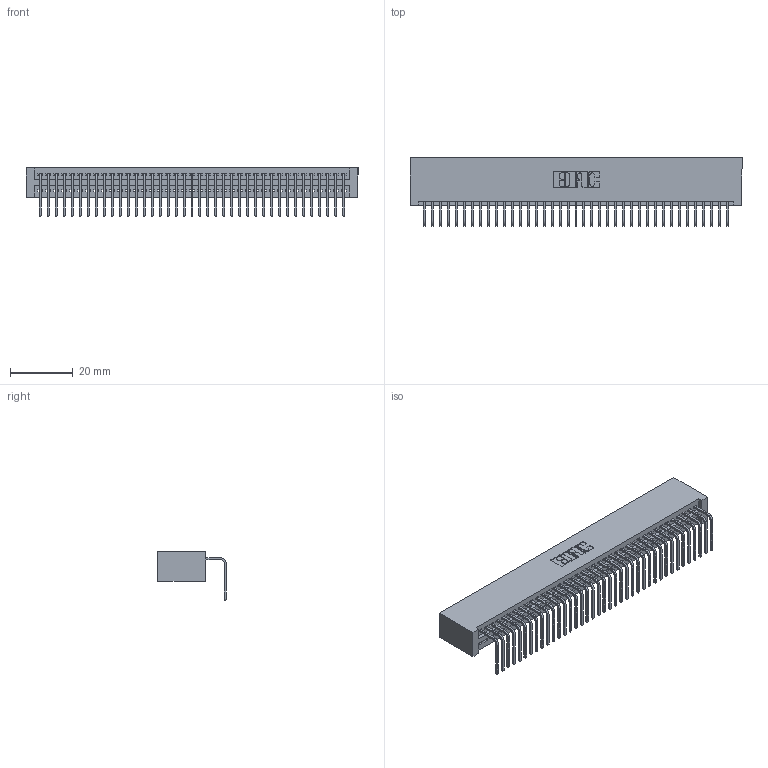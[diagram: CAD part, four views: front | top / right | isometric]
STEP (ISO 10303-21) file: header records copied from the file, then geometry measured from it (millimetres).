
FILE_DESCRIPTION (( 'STEP AP203' ), '1' );
FILE_NAME ('345-039-558-101.STEP', '2019-10-10T15:48:00', ( '' ), ( '' ), 'SwSTEP 2.0', 'SolidWorks 2016', '' );
FILE_SCHEMA (( 'CONFIG_CONTROL_DESIGN' ));
Length unit declared in the file: inch
Products named in the file (3): 345-039-558-101; 345 Part_No Mounting Lugs; 345-292-001_558 Tail - 2
Assembly tree (40 placements, depth 2):
  345-039-558-101
    345 Part_No Mounting Lugs
    345-292-001_558 Tail - 2  x39
Bounding box: 105.66 x 21.83 x 15.37 mm (x, y, z)
Volume: 10725.8 mm3; surface area: 15166.5 mm2
Topology: 40 solids, 40 shells, 2458 faces, 7415 edges, 4890 vertices
Faces by surface type: plane 1714, cylinder 744
Entity records: 29563 total; most frequent: CARTESIAN_POINT 5129, ORIENTED_EDGE 5102, DIRECTION 4477, EDGE_CURVE 2551, VECTOR 2271, LINE 2271, VERTEX_POINT 1698, AXIS2_PLACEMENT_3D 1103
